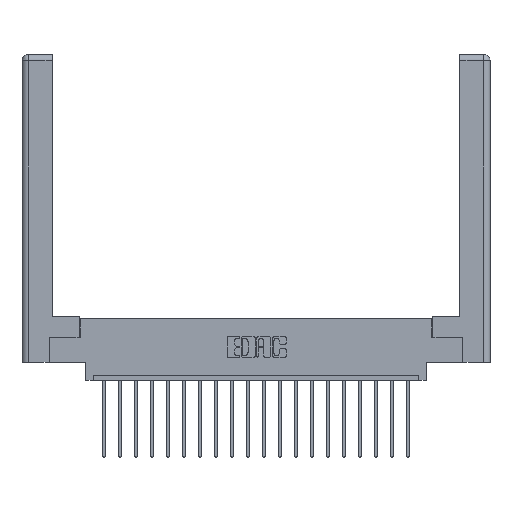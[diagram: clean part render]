
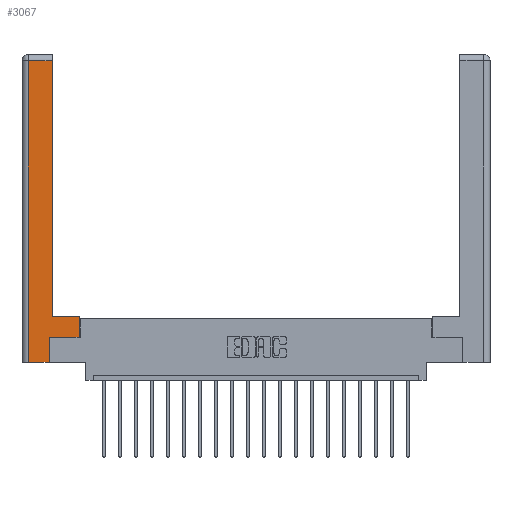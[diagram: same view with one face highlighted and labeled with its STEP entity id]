
A CAD part, top view. The second image highlights one B-rep face of the part: STEP entity #3067.
In plain terms, the highlighted planar face has unit normal (0, 0, 1).
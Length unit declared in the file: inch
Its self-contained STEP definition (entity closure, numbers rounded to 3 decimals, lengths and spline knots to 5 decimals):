
#97 = VERTEX_POINT ( 'NONE', #3081 ) ;
#523 = DIRECTION ( 'NONE',  ( 0., -1., 0. ) ) ;
#802 = CARTESIAN_POINT ( 'NONE',  ( 0.0615, 0., 0. ) ) ;
#1188 = CARTESIAN_POINT ( 'NONE',  ( 0.565, 0.45, 0. ) ) ;
#1220 = LINE ( 'NONE', #2751, #6691 ) ;
#1252 = CARTESIAN_POINT ( 'NONE',  ( 0.265, 0.245, 0. ) ) ;
#1760 = ORIENTED_EDGE ( 'NONE', *, *, #9945, .T. ) ;
#2297 = VECTOR ( 'NONE', #523, 39.37008 ) ;
#2471 = ORIENTED_EDGE ( 'NONE', *, *, #12759, .T. ) ;
#2751 = CARTESIAN_POINT ( 'NONE',  ( 0.265, 0.245, 0. ) ) ;
#3067 = ADVANCED_FACE ( 'NONE', ( #6536 ), #20353, .F. ) ;
#3081 = CARTESIAN_POINT ( 'NONE',  ( 0.0615, 2.94, 0. ) ) ;
#3092 = ORIENTED_EDGE ( 'NONE', *, *, #8662, .T. ) ;
#3508 = ORIENTED_EDGE ( 'NONE', *, *, #16116, .T. ) ;
#3588 = VERTEX_POINT ( 'NONE', #7598 ) ;
#3947 = EDGE_CURVE ( 'NONE', #97, #7323, #8228, .T. ) ;
#4123 = CARTESIAN_POINT ( 'NONE',  ( 0.295, 3., 0. ) ) ;
#4393 = VERTEX_POINT ( 'NONE', #1252 ) ;
#4605 = CARTESIAN_POINT ( 'NONE',  ( 0.265, 0., 0. ) ) ;
#4627 = LINE ( 'NONE', #6872, #15587 ) ;
#5607 = DIRECTION ( 'NONE',  ( 1., 0., 0. ) ) ;
#5729 = VERTEX_POINT ( 'NONE', #6200 ) ;
#5732 = DIRECTION ( 'NONE',  ( 0., 1., 0. ) ) ;
#6137 = ORIENTED_EDGE ( 'NONE', *, *, #13797, .T. ) ;
#6149 = DIRECTION ( 'NONE',  ( 1., 0., 0. ) ) ;
#6200 = CARTESIAN_POINT ( 'NONE',  ( 0.565, 0.245, 0. ) ) ;
#6536 = FACE_OUTER_BOUND ( 'NONE', #9487, .T. ) ;
#6691 = VECTOR ( 'NONE', #9621, 39.37008 ) ;
#6789 = ORIENTED_EDGE ( 'NONE', *, *, #9881, .T. ) ;
#6797 = LINE ( 'NONE', #4605, #20431 ) ;
#6872 = CARTESIAN_POINT ( 'NONE',  ( 0.295, 0.45, 0. ) ) ;
#7276 = LINE ( 'NONE', #17065, #10999 ) ;
#7323 = VERTEX_POINT ( 'NONE', #18235 ) ;
#7598 = CARTESIAN_POINT ( 'NONE',  ( 0.295, 0.45, 0. ) ) ;
#7914 = VERTEX_POINT ( 'NONE', #13718 ) ;
#8225 = ORIENTED_EDGE ( 'NONE', *, *, #18744, .T. ) ;
#8228 = LINE ( 'NONE', #802, #2297 ) ;
#8657 = LINE ( 'NONE', #1188, #15638 ) ;
#8662 = EDGE_CURVE ( 'NONE', #4393, #5729, #11062, .T. ) ;
#9021 = DIRECTION ( 'NONE',  ( 0., 1., 0. ) ) ;
#9487 = EDGE_LOOP ( 'NONE', ( #8225, #6789, #14673, #1760, #3508, #3092, #2471, #6137 ) ) ;
#9621 = DIRECTION ( 'NONE',  ( 0., 1., 0. ) ) ;
#9759 = LINE ( 'NONE', #4123, #13766 ) ;
#9881 = EDGE_CURVE ( 'NONE', #11324, #97, #7276, .T. ) ;
#9945 = EDGE_CURVE ( 'NONE', #7323, #7914, #6797, .T. ) ;
#9956 = CARTESIAN_POINT ( 'NONE',  ( 0.565, 0.245, 0. ) ) ;
#10883 = DIRECTION ( 'NONE',  ( 0., 0., -1. ) ) ;
#10987 = DIRECTION ( 'NONE',  ( -1., 0., 0. ) ) ;
#10999 = VECTOR ( 'NONE', #10987, 39.37008 ) ;
#11062 = LINE ( 'NONE', #9956, #12580 ) ;
#11324 = VERTEX_POINT ( 'NONE', #16647 ) ;
#12580 = VECTOR ( 'NONE', #5607, 39.37008 ) ;
#12759 = EDGE_CURVE ( 'NONE', #5729, #14516, #8657, .T. ) ;
#13273 = DIRECTION ( 'NONE',  ( -1., 0., 0. ) ) ;
#13718 = CARTESIAN_POINT ( 'NONE',  ( 0.265, 0., 0. ) ) ;
#13766 = VECTOR ( 'NONE', #5732, 39.37008 ) ;
#13797 = EDGE_CURVE ( 'NONE', #14516, #3588, #4627, .T. ) ;
#14516 = VERTEX_POINT ( 'NONE', #19661 ) ;
#14673 = ORIENTED_EDGE ( 'NONE', *, *, #3947, .T. ) ;
#15587 = VECTOR ( 'NONE', #13273, 39.37008 ) ;
#15638 = VECTOR ( 'NONE', #9021, 39.37008 ) ;
#16116 = EDGE_CURVE ( 'NONE', #7914, #4393, #1220, .T. ) ;
#16514 = AXIS2_PLACEMENT_3D ( 'NONE', #20417, #10883, #18634 ) ;
#16647 = CARTESIAN_POINT ( 'NONE',  ( 0.295, 2.94, 0. ) ) ;
#17065 = CARTESIAN_POINT ( 'NONE',  ( 0.0615, 2.94, 0. ) ) ;
#18235 = CARTESIAN_POINT ( 'NONE',  ( 0.0615, 0., 0. ) ) ;
#18634 = DIRECTION ( 'NONE',  ( -1., 0., 0. ) ) ;
#18744 = EDGE_CURVE ( 'NONE', #3588, #11324, #9759, .T. ) ;
#19661 = CARTESIAN_POINT ( 'NONE',  ( 0.565, 0.45, 0. ) ) ;
#20353 = PLANE ( 'NONE',  #16514 ) ;
#20417 = CARTESIAN_POINT ( 'NONE',  ( 0., 0., 0. ) ) ;
#20431 = VECTOR ( 'NONE', #6149, 39.37008 ) ;
